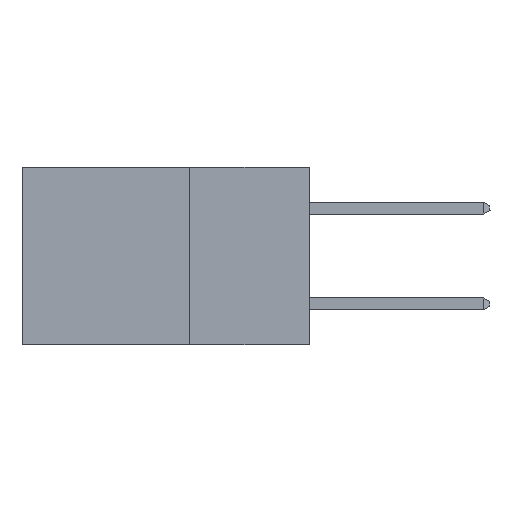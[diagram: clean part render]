
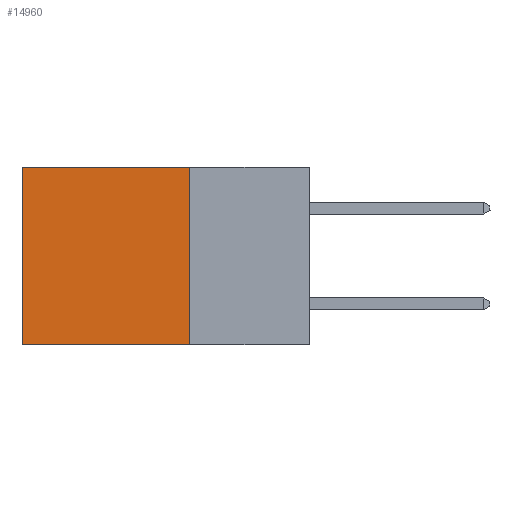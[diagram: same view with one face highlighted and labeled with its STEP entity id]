
A CAD part, left-side view. The second image highlights one B-rep face of the part: STEP entity #14960.
In plain terms, the highlighted planar face has unit normal (-1, 0, 0).
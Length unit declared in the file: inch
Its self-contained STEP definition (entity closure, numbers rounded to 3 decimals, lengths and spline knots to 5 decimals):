
#1905 = EDGE_CURVE ( 'NONE', #13465, #15336, #38141, .T. ) ;
#2610 = CARTESIAN_POINT ( 'NONE',  ( 0.2875, 0.25, 0. ) ) ;
#7622 = VECTOR ( 'NONE', #11207, 39.37008 ) ;
#7887 = VECTOR ( 'NONE', #13303, 39.37008 ) ;
#8583 = LINE ( 'NONE', #2610, #12621 ) ;
#9186 = DIRECTION ( 'NONE',  ( 0., 0., -1. ) ) ;
#9965 = CARTESIAN_POINT ( 'NONE',  ( 0.2875, 0.25, 0. ) ) ;
#10593 = ORIENTED_EDGE ( 'NONE', *, *, #35616, .F. ) ;
#11207 = DIRECTION ( 'NONE',  ( 0., 1., 0. ) ) ;
#11592 = CARTESIAN_POINT ( 'NONE',  ( 0.2875, 0.6, -0.37 ) ) ;
#12607 = CARTESIAN_POINT ( 'NONE',  ( 0.2875, 0.6, 0. ) ) ;
#12621 = VECTOR ( 'NONE', #9186, 39.37008 ) ;
#13005 = VERTEX_POINT ( 'NONE', #20509 ) ;
#13303 = DIRECTION ( 'NONE',  ( 0., 1., 0. ) ) ;
#13465 = VERTEX_POINT ( 'NONE', #39517 ) ;
#14960 = ADVANCED_FACE ( 'NONE', ( #24784 ), #19411, .F. ) ;
#15336 = VERTEX_POINT ( 'NONE', #11592 ) ;
#18144 = EDGE_CURVE ( 'NONE', #13005, #34976, #26826, .T. ) ;
#19011 = DIRECTION ( 'NONE',  ( 1., 0., 0. ) ) ;
#19411 = PLANE ( 'NONE',  #23214 ) ;
#20509 = CARTESIAN_POINT ( 'NONE',  ( 0.2875, 0.25, 0. ) ) ;
#20822 = VECTOR ( 'NONE', #21200, 39.37008 ) ;
#21200 = DIRECTION ( 'NONE',  ( 0., 0., -1. ) ) ;
#21603 = CARTESIAN_POINT ( 'NONE',  ( 0.2875, 0.6, 0. ) ) ;
#23214 = AXIS2_PLACEMENT_3D ( 'NONE', #9965, #19011, #34411 ) ;
#23563 = ORIENTED_EDGE ( 'NONE', *, *, #18144, .T. ) ;
#24784 = FACE_OUTER_BOUND ( 'NONE', #35179, .T. ) ;
#26826 = LINE ( 'NONE', #39322, #7622 ) ;
#28921 = CARTESIAN_POINT ( 'NONE',  ( 0.2875, 0.25, -0.37 ) ) ;
#29042 = ORIENTED_EDGE ( 'NONE', *, *, #39597, .T. ) ;
#32268 = ORIENTED_EDGE ( 'NONE', *, *, #1905, .F. ) ;
#34411 = DIRECTION ( 'NONE',  ( 0., 0., -1. ) ) ;
#34976 = VERTEX_POINT ( 'NONE', #12607 ) ;
#35179 = EDGE_LOOP ( 'NONE', ( #29042, #32268, #10593, #23563 ) ) ;
#35616 = EDGE_CURVE ( 'NONE', #13005, #13465, #8583, .T. ) ;
#38141 = LINE ( 'NONE', #28921, #7887 ) ;
#39322 = CARTESIAN_POINT ( 'NONE',  ( 0.2875, 0.25, 0. ) ) ;
#39517 = CARTESIAN_POINT ( 'NONE',  ( 0.2875, 0.25, -0.37 ) ) ;
#39597 = EDGE_CURVE ( 'NONE', #34976, #15336, #40258, .T. ) ;
#40258 = LINE ( 'NONE', #21603, #20822 ) ;
